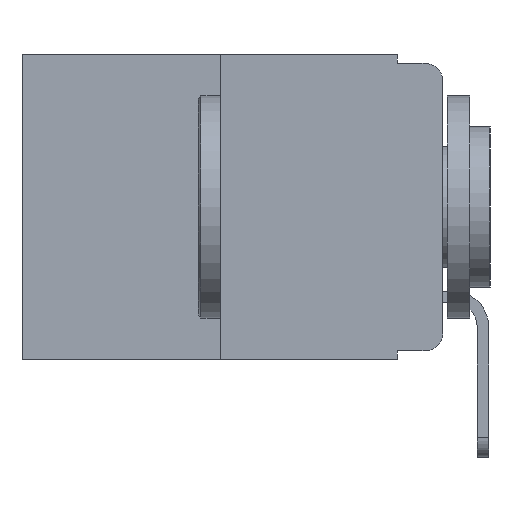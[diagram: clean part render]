
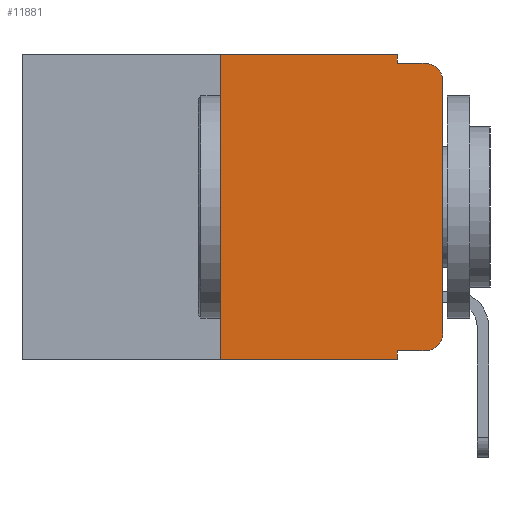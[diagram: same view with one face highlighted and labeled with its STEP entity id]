
A CAD part, left-side view. The second image highlights one B-rep face of the part: STEP entity #11881.
In plain terms, the highlighted planar face has unit normal (-1, 0, 0).
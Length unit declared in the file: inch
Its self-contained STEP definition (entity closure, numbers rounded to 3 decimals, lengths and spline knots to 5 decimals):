
#324 = VECTOR ( 'NONE', #13102, 39.37008 ) ;
#817 = VERTEX_POINT ( 'NONE', #854 ) ;
#854 = CARTESIAN_POINT ( 'NONE',  ( 0., 0.25, -0.343 ) ) ;
#1207 = CARTESIAN_POINT ( 'NONE',  ( 0., 0.051, 0. ) ) ;
#1419 = VERTEX_POINT ( 'NONE', #17080 ) ;
#1529 = DIRECTION ( 'NONE',  ( 0., -1., 0. ) ) ;
#1642 = CARTESIAN_POINT ( 'NONE',  ( 0., 0.051, -0.343 ) ) ;
#1679 = DIRECTION ( 'NONE',  ( 0., -1., 0. ) ) ;
#2909 = VERTEX_POINT ( 'NONE', #6928 ) ;
#3010 = VECTOR ( 'NONE', #13276, 39.37008 ) ;
#3628 = VERTEX_POINT ( 'NONE', #18003 ) ;
#3725 = AXIS2_PLACEMENT_3D ( 'NONE', #13928, #15175, #7265 ) ;
#4147 = PLANE ( 'NONE',  #3725 ) ;
#4203 = VECTOR ( 'NONE', #1529, 39.37008 ) ;
#4470 = CARTESIAN_POINT ( 'NONE',  ( 0., 0.473, 0. ) ) ;
#4690 = CIRCLE ( 'NONE', #9109, 0.02 ) ;
#4710 = CARTESIAN_POINT ( 'NONE',  ( 0., 0.25, 0. ) ) ;
#4741 = ORIENTED_EDGE ( 'NONE', *, *, #9117, .F. ) ;
#4777 = CARTESIAN_POINT ( 'NONE',  ( 0., 0.051, -0.333 ) ) ;
#4984 = ORIENTED_EDGE ( 'NONE', *, *, #8375, .T. ) ;
#5002 = ORIENTED_EDGE ( 'NONE', *, *, #9095, .F. ) ;
#5113 = ORIENTED_EDGE ( 'NONE', *, *, #7750, .F. ) ;
#5141 = CARTESIAN_POINT ( 'NONE',  ( 0., 0.051, -0.333 ) ) ;
#5178 = VECTOR ( 'NONE', #9305, 39.37008 ) ;
#5288 = ORIENTED_EDGE ( 'NONE', *, *, #9093, .F. ) ;
#5405 = ORIENTED_EDGE ( 'NONE', *, *, #9087, .F. ) ;
#6015 = CARTESIAN_POINT ( 'NONE',  ( 0., 0., -0.03 ) ) ;
#6016 = DIRECTION ( 'NONE',  ( 0., -1., 0. ) ) ;
#6258 = DIRECTION ( 'NONE',  ( 0., 0., 1. ) ) ;
#6386 = DIRECTION ( 'NONE',  ( -1., 0., 0. ) ) ;
#6746 = VERTEX_POINT ( 'NONE', #10808 ) ;
#6928 = CARTESIAN_POINT ( 'NONE',  ( 0., 0.02, -0.333 ) ) ;
#6984 = VERTEX_POINT ( 'NONE', #13766 ) ;
#7265 = DIRECTION ( 'NONE',  ( 0., 0., -1. ) ) ;
#7325 = VERTEX_POINT ( 'NONE', #1642 ) ;
#7622 = LINE ( 'NONE', #7918, #3010 ) ;
#7748 = CARTESIAN_POINT ( 'NONE',  ( 0., 0.02, -0.03 ) ) ;
#7750 = EDGE_CURVE ( 'NONE', #6746, #9989, #13313, .T. ) ;
#7820 = CARTESIAN_POINT ( 'NONE',  ( 0., 0.051, 0. ) ) ;
#7918 = CARTESIAN_POINT ( 'NONE',  ( 0., 0.473, -0.343 ) ) ;
#8313 = ORIENTED_EDGE ( 'NONE', *, *, #9152, .T. ) ;
#8326 = LINE ( 'NONE', #14320, #4203 ) ;
#8375 = EDGE_CURVE ( 'NONE', #817, #7325, #7622, .T. ) ;
#8614 = ORIENTED_EDGE ( 'NONE', *, *, #9150, .T. ) ;
#9060 = EDGE_CURVE ( 'NONE', #6984, #15531, #12680, .T. ) ;
#9063 = EDGE_CURVE ( 'NONE', #15531, #3628, #4690, .T. ) ;
#9087 = EDGE_CURVE ( 'NONE', #1419, #3628, #8326, .T. ) ;
#9093 = EDGE_CURVE ( 'NONE', #9989, #1419, #15191, .T. ) ;
#9095 = EDGE_CURVE ( 'NONE', #817, #6746, #17983, .T. ) ;
#9109 = AXIS2_PLACEMENT_3D ( 'NONE', #7748, #16733, #9247 ) ;
#9117 = EDGE_CURVE ( 'NONE', #13322, #7325, #14791, .T. ) ;
#9150 = EDGE_CURVE ( 'NONE', #13322, #2909, #14020, .T. ) ;
#9152 = EDGE_CURVE ( 'NONE', #2909, #6984, #17239, .T. ) ;
#9247 = DIRECTION ( 'NONE',  ( 0., 0., -1. ) ) ;
#9305 = DIRECTION ( 'NONE',  ( 0., 0., -1. ) ) ;
#9408 = FACE_OUTER_BOUND ( 'NONE', #11925, .T. ) ;
#9639 = ORIENTED_EDGE ( 'NONE', *, *, #9060, .T. ) ;
#9745 = ORIENTED_EDGE ( 'NONE', *, *, #9063, .T. ) ;
#9919 = VECTOR ( 'NONE', #6016, 39.37008 ) ;
#9989 = VERTEX_POINT ( 'NONE', #1207 ) ;
#10689 = VECTOR ( 'NONE', #1679, 39.37008 ) ;
#10808 = CARTESIAN_POINT ( 'NONE',  ( 0., 0.25, 0. ) ) ;
#11476 = VECTOR ( 'NONE', #6258, 39.37008 ) ;
#11813 = CARTESIAN_POINT ( 'NONE',  ( 0., 0., 0. ) ) ;
#11864 = CARTESIAN_POINT ( 'NONE',  ( 0., 0.051, 0. ) ) ;
#11876 = VECTOR ( 'NONE', #17942, 39.37008 ) ;
#11881 = ADVANCED_FACE ( 'NONE', ( #9408 ), #4147, .F. ) ;
#11925 = EDGE_LOOP ( 'NONE', ( #9639, #9745, #5405, #5288, #5113, #5002, #4984, #4741, #8614, #8313 ) ) ;
#12680 = LINE ( 'NONE', #11813, #324 ) ;
#13102 = DIRECTION ( 'NONE',  ( 0., 0., 1. ) ) ;
#13276 = DIRECTION ( 'NONE',  ( 0., -1., 0. ) ) ;
#13313 = LINE ( 'NONE', #4470, #9919 ) ;
#13322 = VERTEX_POINT ( 'NONE', #5141 ) ;
#13766 = CARTESIAN_POINT ( 'NONE',  ( 0., 0., -0.313 ) ) ;
#13928 = CARTESIAN_POINT ( 'NONE',  ( 0., 0.473, 0. ) ) ;
#14020 = LINE ( 'NONE', #4777, #10689 ) ;
#14259 = AXIS2_PLACEMENT_3D ( 'NONE', #14467, #6386, #15708 ) ;
#14320 = CARTESIAN_POINT ( 'NONE',  ( 0., 0.051, -0.01 ) ) ;
#14467 = CARTESIAN_POINT ( 'NONE',  ( 0., 0.02, -0.313 ) ) ;
#14791 = LINE ( 'NONE', #7820, #5178 ) ;
#15175 = DIRECTION ( 'NONE',  ( 1., 0., 0. ) ) ;
#15191 = LINE ( 'NONE', #11864, #11876 ) ;
#15531 = VERTEX_POINT ( 'NONE', #6015 ) ;
#15708 = DIRECTION ( 'NONE',  ( 0., 0., -1. ) ) ;
#16733 = DIRECTION ( 'NONE',  ( -1., 0., 0. ) ) ;
#17080 = CARTESIAN_POINT ( 'NONE',  ( 0., 0.051, -0.01 ) ) ;
#17239 = CIRCLE ( 'NONE', #14259, 0.02 ) ;
#17942 = DIRECTION ( 'NONE',  ( 0., 0., -1. ) ) ;
#17983 = LINE ( 'NONE', #4710, #11476 ) ;
#18003 = CARTESIAN_POINT ( 'NONE',  ( 0., 0.02, -0.01 ) ) ;
